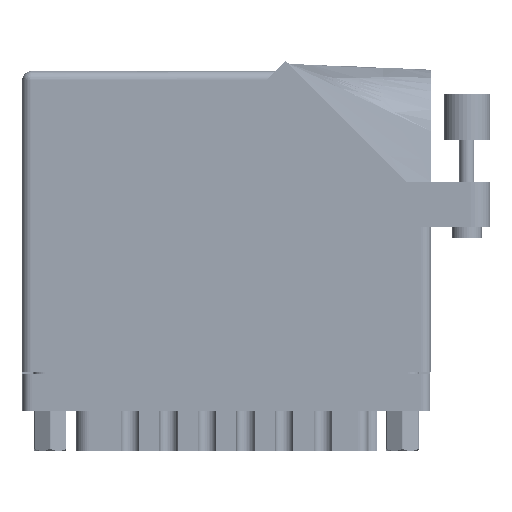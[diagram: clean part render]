
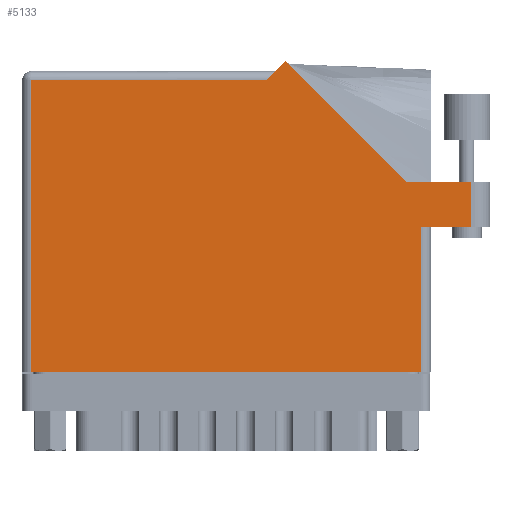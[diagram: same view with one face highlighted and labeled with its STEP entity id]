
A CAD part, front view. The second image highlights one B-rep face of the part: STEP entity #5133.
In plain terms, the highlighted face is planar.
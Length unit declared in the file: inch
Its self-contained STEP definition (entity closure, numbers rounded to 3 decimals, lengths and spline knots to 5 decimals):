
#1261 = VECTOR ( 'NONE', #88094, 39.37008 ) ;
#4424 = CARTESIAN_POINT ( 'NONE',  ( 0.062, 1.968, 0. ) ) ;
#5133 = ADVANCED_FACE ( 'NONE', ( #28216 ), #21301, .F. ) ;
#5143 = CARTESIAN_POINT ( 'NONE',  ( 0.062, 0., 0. ) ) ;
#5210 = DIRECTION ( 'NONE',  ( -1., 0., 0. ) ) ;
#6509 = CARTESIAN_POINT ( 'NONE',  ( 2.755, 0.98, 0. ) ) ;
#7330 = VECTOR ( 'NONE', #64570, 39.37008 ) ;
#7682 = CARTESIAN_POINT ( 'NONE',  ( 0., 1.968, 0. ) ) ;
#9017 = ORIENTED_EDGE ( 'NONE', *, *, #64613, .T. ) ;
#10859 = LINE ( 'NONE', #5143, #95363 ) ;
#10976 = EDGE_CURVE ( 'NONE', #39885, #70539, #38225, .T. ) ;
#11881 = EDGE_CURVE ( 'NONE', #32259, #66170, #52070, .T. ) ;
#13618 = DIRECTION ( 'NONE',  ( -0.707, -0.707, 0. ) ) ;
#17389 = ORIENTED_EDGE ( 'NONE', *, *, #10976, .T. ) ;
#18750 = VERTEX_POINT ( 'NONE', #4424 ) ;
#21301 = PLANE ( 'NONE',  #90622 ) ;
#21896 = LINE ( 'NONE', #58687, #73127 ) ;
#22709 = DIRECTION ( 'NONE',  ( 0., 0., -1. ) ) ;
#25158 = CARTESIAN_POINT ( 'NONE',  ( 3.03, 1.287, 0. ) ) ;
#27834 = VECTOR ( 'NONE', #92121, 39.37008 ) ;
#27947 = VERTEX_POINT ( 'NONE', #51259 ) ;
#28042 = VECTOR ( 'NONE', #70169, 39.37008 ) ;
#28216 = FACE_OUTER_BOUND ( 'NONE', #58131, .T. ) ;
#29363 = LINE ( 'NONE', #86220, #69016 ) ;
#31073 = CARTESIAN_POINT ( 'NONE',  ( 3.03, 0.98, 0. ) ) ;
#32259 = VERTEX_POINT ( 'NONE', #31073 ) ;
#38042 = DIRECTION ( 'NONE',  ( 0., -1., 0. ) ) ;
#38225 = LINE ( 'NONE', #63017, #28042 ) ;
#39885 = VERTEX_POINT ( 'NONE', #42876 ) ;
#40045 = VERTEX_POINT ( 'NONE', #75799 ) ;
#42876 = CARTESIAN_POINT ( 'NONE',  ( 0.062, 0., 0. ) ) ;
#43821 = EDGE_CURVE ( 'NONE', #40045, #32259, #69172, .T. ) ;
#44569 = EDGE_CURVE ( 'NONE', #27947, #18750, #52312, .T. ) ;
#49348 = EDGE_CURVE ( 'NONE', #93440, #98027, #21896, .T. ) ;
#51195 = DIRECTION ( 'NONE',  ( -0.707, 0.707, 0. ) ) ;
#51259 = CARTESIAN_POINT ( 'NONE',  ( 1.643, 1.968, 0. ) ) ;
#51886 = DIRECTION ( 'NONE',  ( -1., 0., 0. ) ) ;
#52070 = LINE ( 'NONE', #57026, #7330 ) ;
#52312 = LINE ( 'NONE', #7682, #56231 ) ;
#53470 = ORIENTED_EDGE ( 'NONE', *, *, #44569, .T. ) ;
#56231 = VECTOR ( 'NONE', #98171, 39.37008 ) ;
#57026 = CARTESIAN_POINT ( 'NONE',  ( 3.03, 1.287, 0. ) ) ;
#58131 = EDGE_LOOP ( 'NONE', ( #102337, #95791, #100486, #95651, #62114, #53470, #58550, #17389, #9017 ) ) ;
#58550 = ORIENTED_EDGE ( 'NONE', *, *, #87517, .T. ) ;
#58687 = CARTESIAN_POINT ( 'NONE',  ( 2.58942, 1.287, 0. ) ) ;
#62078 = CARTESIAN_POINT ( 'NONE',  ( 0., 2.03, 0. ) ) ;
#62114 = ORIENTED_EDGE ( 'NONE', *, *, #68123, .T. ) ;
#63017 = CARTESIAN_POINT ( 'NONE',  ( 0., 0., 0. ) ) ;
#64570 = DIRECTION ( 'NONE',  ( 0., 1., 0. ) ) ;
#64613 = EDGE_CURVE ( 'NONE', #70539, #40045, #93198, .T. ) ;
#66170 = VERTEX_POINT ( 'NONE', #25158 ) ;
#68123 = EDGE_CURVE ( 'NONE', #98027, #27947, #29363, .T. ) ;
#69016 = VECTOR ( 'NONE', #13618, 39.37008 ) ;
#69172 = LINE ( 'NONE', #6509, #1261 ) ;
#70169 = DIRECTION ( 'NONE',  ( 1., 0., 0. ) ) ;
#70539 = VERTEX_POINT ( 'NONE', #76502 ) ;
#73127 = VECTOR ( 'NONE', #51195, 39.37008 ) ;
#75799 = CARTESIAN_POINT ( 'NONE',  ( 2.693, 0.98, 0. ) ) ;
#76502 = CARTESIAN_POINT ( 'NONE',  ( 2.693, 0., 0. ) ) ;
#76598 = CARTESIAN_POINT ( 'NONE',  ( 3.155, 1.287, 0. ) ) ;
#77283 = VECTOR ( 'NONE', #51886, 39.37008 ) ;
#82819 = CARTESIAN_POINT ( 'NONE',  ( 2.693, 0.98, 0. ) ) ;
#84468 = CARTESIAN_POINT ( 'NONE',  ( 2.58942, 1.287, 0. ) ) ;
#86220 = CARTESIAN_POINT ( 'NONE',  ( 1.705, 2.03, 0. ) ) ;
#87517 = EDGE_CURVE ( 'NONE', #18750, #39885, #10859, .T. ) ;
#87927 = EDGE_CURVE ( 'NONE', #66170, #93440, #92619, .T. ) ;
#88094 = DIRECTION ( 'NONE',  ( 1., 0., 0. ) ) ;
#90622 = AXIS2_PLACEMENT_3D ( 'NONE', #62078, #22709, #5210 ) ;
#92121 = DIRECTION ( 'NONE',  ( 0., 1., 0. ) ) ;
#92619 = LINE ( 'NONE', #76598, #77283 ) ;
#93198 = LINE ( 'NONE', #82819, #27834 ) ;
#93440 = VERTEX_POINT ( 'NONE', #84468 ) ;
#95363 = VECTOR ( 'NONE', #38042, 39.37008 ) ;
#95651 = ORIENTED_EDGE ( 'NONE', *, *, #49348, .T. ) ;
#95791 = ORIENTED_EDGE ( 'NONE', *, *, #11881, .T. ) ;
#98027 = VERTEX_POINT ( 'NONE', #103716 ) ;
#98171 = DIRECTION ( 'NONE',  ( -1., 0., 0. ) ) ;
#100486 = ORIENTED_EDGE ( 'NONE', *, *, #87927, .T. ) ;
#102337 = ORIENTED_EDGE ( 'NONE', *, *, #43821, .T. ) ;
#103716 = CARTESIAN_POINT ( 'NONE',  ( 1.77571, 2.10071, 0. ) ) ;
